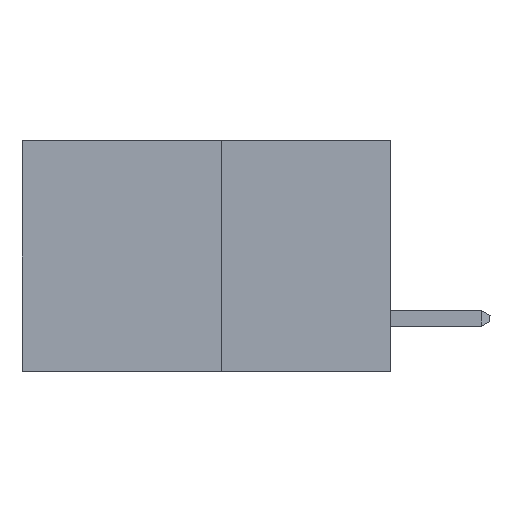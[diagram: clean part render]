
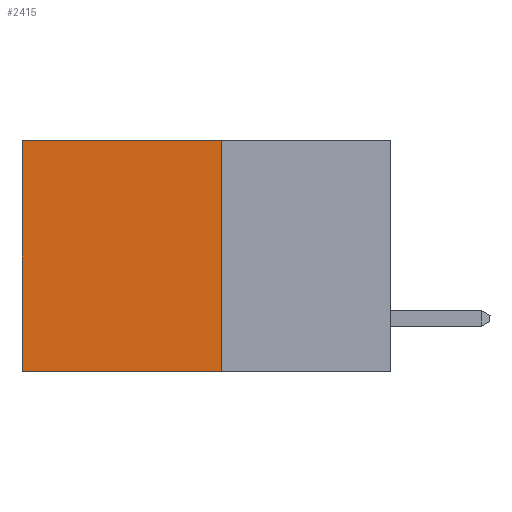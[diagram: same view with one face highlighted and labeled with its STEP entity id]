
A CAD part, left-side view. The second image highlights one B-rep face of the part: STEP entity #2415.
In plain terms, the highlighted planar face has unit normal (-1, 0, 0).
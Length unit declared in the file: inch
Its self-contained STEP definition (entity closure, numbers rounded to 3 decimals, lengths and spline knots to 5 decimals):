
#1022 = DIRECTION ( 'NONE',  ( 0., 0., -1. ) ) ;
#1087 = DIRECTION ( 'NONE',  ( 1., 0., 0. ) ) ;
#1264 = PLANE ( 'NONE',  #23041 ) ;
#2400 = CARTESIAN_POINT ( 'NONE',  ( 0.277, 0.27, -0.37 ) ) ;
#2415 = ADVANCED_FACE ( 'NONE', ( #17130 ), #1264, .F. ) ;
#2440 = CARTESIAN_POINT ( 'NONE',  ( 0.277, 0.27, -0.37 ) ) ;
#4108 = ORIENTED_EDGE ( 'NONE', *, *, #24584, .F. ) ;
#5136 = VERTEX_POINT ( 'NONE', #26682 ) ;
#5758 = LINE ( 'NONE', #12507, #12672 ) ;
#7052 = EDGE_CURVE ( 'NONE', #5136, #25456, #23789, .T. ) ;
#8861 = EDGE_LOOP ( 'NONE', ( #27829, #4108, #27506, #27787 ) ) ;
#9184 = VERTEX_POINT ( 'NONE', #13155 ) ;
#11054 = EDGE_CURVE ( 'NONE', #9184, #28934, #29944, .T. ) ;
#11223 = DIRECTION ( 'NONE',  ( 0., 0., -1. ) ) ;
#12507 = CARTESIAN_POINT ( 'NONE',  ( 0.277, 0.27, 0. ) ) ;
#12672 = VECTOR ( 'NONE', #28556, 39.37008 ) ;
#13155 = CARTESIAN_POINT ( 'NONE',  ( 0.277, 0.27, 0. ) ) ;
#14074 = LINE ( 'NONE', #2440, #20210 ) ;
#15886 = CARTESIAN_POINT ( 'NONE',  ( 0.277, 0.59, -0.37 ) ) ;
#17003 = CARTESIAN_POINT ( 'NONE',  ( 0.277, 0.27, -0.37 ) ) ;
#17058 = EDGE_CURVE ( 'NONE', #9184, #5136, #5758, .T. ) ;
#17130 = FACE_OUTER_BOUND ( 'NONE', #8861, .T. ) ;
#17738 = VECTOR ( 'NONE', #11223, 39.37008 ) ;
#17822 = VECTOR ( 'NONE', #24416, 39.37008 ) ;
#20210 = VECTOR ( 'NONE', #21089, 39.37008 ) ;
#21089 = DIRECTION ( 'NONE',  ( 0., 1., 0. ) ) ;
#22092 = CARTESIAN_POINT ( 'NONE',  ( 0.277, 0.27, -0.37 ) ) ;
#22338 = CARTESIAN_POINT ( 'NONE',  ( 0.277, 0.59, -0.37 ) ) ;
#23041 = AXIS2_PLACEMENT_3D ( 'NONE', #2400, #1087, #1022 ) ;
#23789 = LINE ( 'NONE', #15886, #17738 ) ;
#24416 = DIRECTION ( 'NONE',  ( 0., 0., -1. ) ) ;
#24584 = EDGE_CURVE ( 'NONE', #28934, #25456, #14074, .T. ) ;
#25456 = VERTEX_POINT ( 'NONE', #22338 ) ;
#26682 = CARTESIAN_POINT ( 'NONE',  ( 0.277, 0.59, 0. ) ) ;
#27506 = ORIENTED_EDGE ( 'NONE', *, *, #11054, .F. ) ;
#27787 = ORIENTED_EDGE ( 'NONE', *, *, #17058, .T. ) ;
#27829 = ORIENTED_EDGE ( 'NONE', *, *, #7052, .T. ) ;
#28556 = DIRECTION ( 'NONE',  ( 0., 1., 0. ) ) ;
#28934 = VERTEX_POINT ( 'NONE', #17003 ) ;
#29944 = LINE ( 'NONE', #22092, #17822 ) ;
